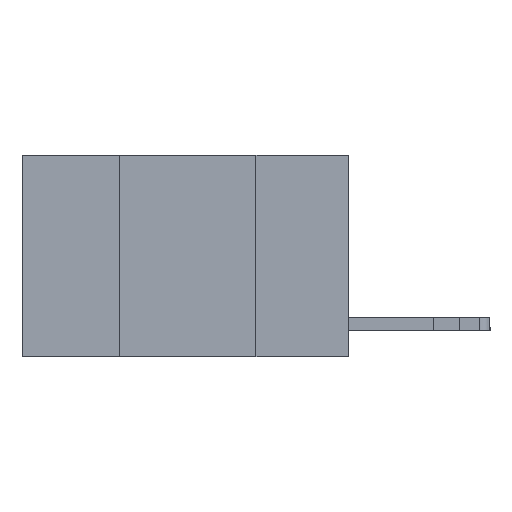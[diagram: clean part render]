
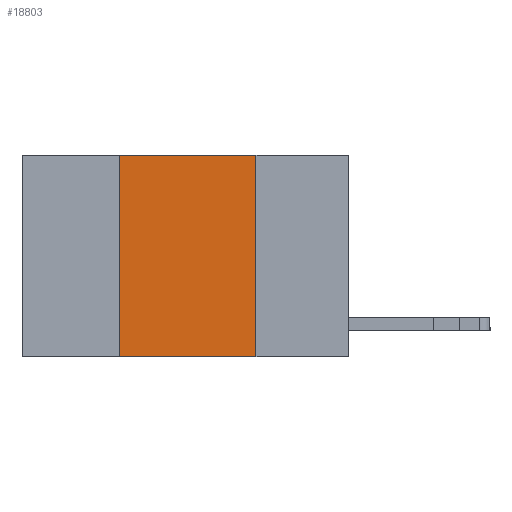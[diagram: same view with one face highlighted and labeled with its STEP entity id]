
A CAD part, left-side view. The second image highlights one B-rep face of the part: STEP entity #18803.
In plain terms, the highlighted planar face has unit normal (-1, 0, 0).
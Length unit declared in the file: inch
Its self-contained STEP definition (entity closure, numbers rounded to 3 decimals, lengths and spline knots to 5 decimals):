
#98 = EDGE_CURVE ( 'NONE', #17639, #9961, #2178, .T. ) ;
#197 = DIRECTION ( 'NONE',  ( 0., -1., 0. ) ) ;
#713 = LINE ( 'NONE', #13669, #15839 ) ;
#1588 = CARTESIAN_POINT ( 'NONE',  ( 0., 0.17, 0. ) ) ;
#2178 = LINE ( 'NONE', #13703, #10264 ) ;
#2278 = DIRECTION ( 'NONE',  ( 0., -1., 0. ) ) ;
#2438 = CARTESIAN_POINT ( 'NONE',  ( 0., 0.17, 0. ) ) ;
#3289 = CARTESIAN_POINT ( 'NONE',  ( 0., 0.17, -0.37 ) ) ;
#3663 = VECTOR ( 'NONE', #197, 39.37008 ) ;
#6098 = CARTESIAN_POINT ( 'NONE',  ( 0., 0.6, 0. ) ) ;
#7115 = ORIENTED_EDGE ( 'NONE', *, *, #11834, .T. ) ;
#7396 = DIRECTION ( 'NONE',  ( 0., 0., -1. ) ) ;
#7429 = DIRECTION ( 'NONE',  ( 1., 0., 0. ) ) ;
#8865 = ORIENTED_EDGE ( 'NONE', *, *, #11651, .F. ) ;
#9031 = EDGE_CURVE ( 'NONE', #9961, #9799, #9965, .T. ) ;
#9136 = LINE ( 'NONE', #17847, #3663 ) ;
#9799 = VERTEX_POINT ( 'NONE', #3289 ) ;
#9961 = VERTEX_POINT ( 'NONE', #2438 ) ;
#9965 = LINE ( 'NONE', #1588, #15115 ) ;
#10264 = VECTOR ( 'NONE', #2278, 39.37008 ) ;
#11463 = ORIENTED_EDGE ( 'NONE', *, *, #98, .F. ) ;
#11651 = EDGE_CURVE ( 'NONE', #18349, #17639, #713, .T. ) ;
#11834 = EDGE_CURVE ( 'NONE', #18349, #9799, #9136, .T. ) ;
#11876 = CARTESIAN_POINT ( 'NONE',  ( 0., 0.42, 0. ) ) ;
#11915 = PLANE ( 'NONE',  #16909 ) ;
#12017 = DIRECTION ( 'NONE',  ( 0., 0., -1. ) ) ;
#12344 = DIRECTION ( 'NONE',  ( 0., 0., 1. ) ) ;
#13669 = CARTESIAN_POINT ( 'NONE',  ( 0., 0.42, 0. ) ) ;
#13703 = CARTESIAN_POINT ( 'NONE',  ( 0., 0.6, 0. ) ) ;
#15115 = VECTOR ( 'NONE', #7396, 39.37008 ) ;
#15408 = EDGE_LOOP ( 'NONE', ( #16164, #11463, #8865, #7115 ) ) ;
#15839 = VECTOR ( 'NONE', #12344, 39.37008 ) ;
#16164 = ORIENTED_EDGE ( 'NONE', *, *, #9031, .F. ) ;
#16212 = FACE_OUTER_BOUND ( 'NONE', #15408, .T. ) ;
#16909 = AXIS2_PLACEMENT_3D ( 'NONE', #6098, #7429, #12017 ) ;
#17639 = VERTEX_POINT ( 'NONE', #11876 ) ;
#17847 = CARTESIAN_POINT ( 'NONE',  ( 0., 0.6, -0.37 ) ) ;
#17953 = CARTESIAN_POINT ( 'NONE',  ( 0., 0.42, -0.37 ) ) ;
#18349 = VERTEX_POINT ( 'NONE', #17953 ) ;
#18803 = ADVANCED_FACE ( 'NONE', ( #16212 ), #11915, .F. ) ;
